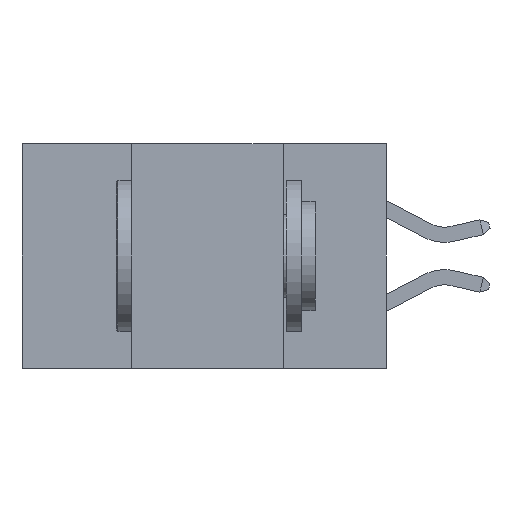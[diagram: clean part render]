
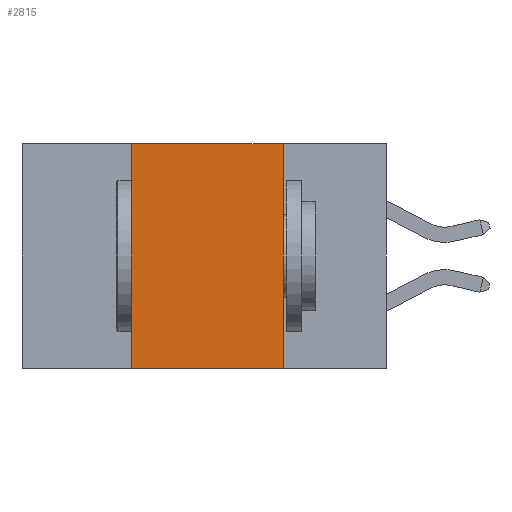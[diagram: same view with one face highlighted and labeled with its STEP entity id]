
A CAD part, left-side view. The second image highlights one B-rep face of the part: STEP entity #2815.
In plain terms, the highlighted planar face has unit normal (-1, 0, 0).
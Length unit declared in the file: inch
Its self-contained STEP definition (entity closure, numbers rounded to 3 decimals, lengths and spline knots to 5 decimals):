
#479 = DIRECTION ( 'NONE',  ( 0., 0., -1. ) ) ;
#923 = EDGE_LOOP ( 'NONE', ( #14987, #11279, #10924, #1330 ) ) ;
#1081 = FACE_OUTER_BOUND ( 'NONE', #923, .T. ) ;
#1215 = CARTESIAN_POINT ( 'NONE',  ( 0., 0.17, 0. ) ) ;
#1330 = ORIENTED_EDGE ( 'NONE', *, *, #12123, .T. ) ;
#1617 = EDGE_CURVE ( 'NONE', #5782, #12479, #17772, .T. ) ;
#1919 = CARTESIAN_POINT ( 'NONE',  ( 0., 0.6, -0.37 ) ) ;
#2138 = LINE ( 'NONE', #1919, #13633 ) ;
#2707 = CARTESIAN_POINT ( 'NONE',  ( 0., 0.42, 0. ) ) ;
#2815 = ADVANCED_FACE ( 'NONE', ( #1081 ), #15914, .F. ) ;
#2908 = VERTEX_POINT ( 'NONE', #12534 ) ;
#5782 = VERTEX_POINT ( 'NONE', #10416 ) ;
#7808 = EDGE_CURVE ( 'NONE', #2908, #10704, #8605, .T. ) ;
#8605 = LINE ( 'NONE', #1215, #15954 ) ;
#8975 = CARTESIAN_POINT ( 'NONE',  ( 0., 0.42, 0. ) ) ;
#9035 = EDGE_CURVE ( 'NONE', #12479, #2908, #10414, .T. ) ;
#9532 = DIRECTION ( 'NONE',  ( 0., -1., 0. ) ) ;
#9994 = VECTOR ( 'NONE', #19221, 39.37008 ) ;
#10414 = LINE ( 'NONE', #18112, #18647 ) ;
#10416 = CARTESIAN_POINT ( 'NONE',  ( 0., 0.42, -0.37 ) ) ;
#10704 = VERTEX_POINT ( 'NONE', #17790 ) ;
#10924 = ORIENTED_EDGE ( 'NONE', *, *, #1617, .F. ) ;
#11279 = ORIENTED_EDGE ( 'NONE', *, *, #9035, .F. ) ;
#12008 = DIRECTION ( 'NONE',  ( 0., 0., -1. ) ) ;
#12123 = EDGE_CURVE ( 'NONE', #5782, #10704, #2138, .T. ) ;
#12479 = VERTEX_POINT ( 'NONE', #2707 ) ;
#12534 = CARTESIAN_POINT ( 'NONE',  ( 0., 0.17, 0. ) ) ;
#13633 = VECTOR ( 'NONE', #9532, 39.37008 ) ;
#14987 = ORIENTED_EDGE ( 'NONE', *, *, #7808, .F. ) ;
#15897 = DIRECTION ( 'NONE',  ( 1., 0., 0. ) ) ;
#15914 = PLANE ( 'NONE',  #16723 ) ;
#15954 = VECTOR ( 'NONE', #479, 39.37008 ) ;
#16723 = AXIS2_PLACEMENT_3D ( 'NONE', #18601, #15897, #12008 ) ;
#17772 = LINE ( 'NONE', #8975, #9994 ) ;
#17790 = CARTESIAN_POINT ( 'NONE',  ( 0., 0.17, -0.37 ) ) ;
#18073 = DIRECTION ( 'NONE',  ( 0., -1., 0. ) ) ;
#18112 = CARTESIAN_POINT ( 'NONE',  ( 0., 0.6, 0. ) ) ;
#18601 = CARTESIAN_POINT ( 'NONE',  ( 0., 0.6, 0. ) ) ;
#18647 = VECTOR ( 'NONE', #18073, 39.37008 ) ;
#19221 = DIRECTION ( 'NONE',  ( 0., 0., 1. ) ) ;
